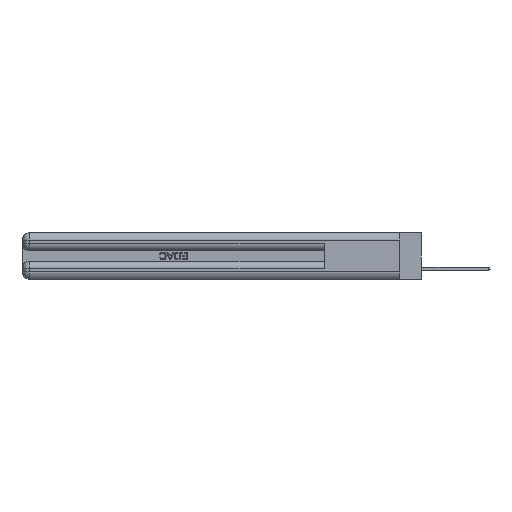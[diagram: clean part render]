
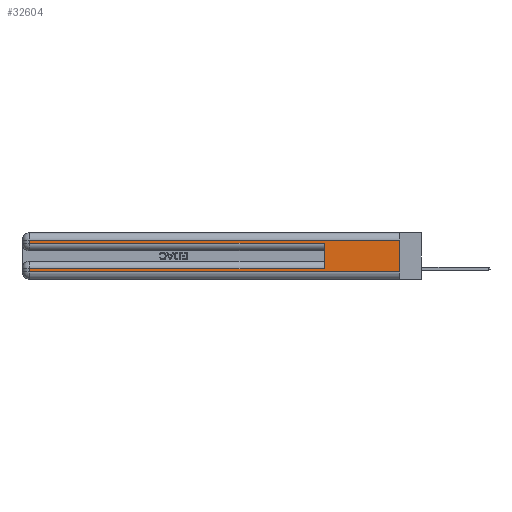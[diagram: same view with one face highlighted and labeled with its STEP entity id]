
A CAD part, left-side view. The second image highlights one B-rep face of the part: STEP entity #32604.
In plain terms, the highlighted planar face has unit normal (-1, 0, 0).
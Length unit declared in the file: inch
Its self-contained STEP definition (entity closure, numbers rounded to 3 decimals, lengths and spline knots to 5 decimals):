
#345 = ORIENTED_EDGE ( 'NONE', *, *, #15838, .F. ) ;
#2131 = CARTESIAN_POINT ( 'NONE',  ( 0., 0., 0.31 ) ) ;
#2187 = DIRECTION ( 'NONE',  ( 0., 0., 1. ) ) ;
#2577 = LINE ( 'NONE', #20068, #21641 ) ;
#3055 = VECTOR ( 'NONE', #5408, 39.37008 ) ;
#3238 = VECTOR ( 'NONE', #14824, 39.37008 ) ;
#3482 = EDGE_CURVE ( 'NONE', #24509, #18671, #12868, .T. ) ;
#3829 = LINE ( 'NONE', #23897, #10947 ) ;
#4015 = DIRECTION ( 'NONE',  ( 0., 0., -1. ) ) ;
#5408 = DIRECTION ( 'NONE',  ( 0., -1., 0. ) ) ;
#6729 = AXIS2_PLACEMENT_3D ( 'NONE', #31331, #17486, #4015 ) ;
#7187 = VERTEX_POINT ( 'NONE', #2131 ) ;
#7640 = CARTESIAN_POINT ( 'NONE',  ( 0., 2.94, 0.31 ) ) ;
#7705 = CARTESIAN_POINT ( 'NONE',  ( 0., 0., 0.085 ) ) ;
#7799 = ORIENTED_EDGE ( 'NONE', *, *, #21911, .F. ) ;
#8224 = CARTESIAN_POINT ( 'NONE',  ( 0., 0., 0.31 ) ) ;
#8374 = VECTOR ( 'NONE', #11844, 39.37008 ) ;
#8451 = EDGE_CURVE ( 'NONE', #42391, #24509, #31142, .T. ) ;
#8482 = DIRECTION ( 'NONE',  ( 0., 1., 0. ) ) ;
#8803 = EDGE_CURVE ( 'NONE', #11566, #16770, #3829, .T. ) ;
#9508 = LINE ( 'NONE', #8224, #8374 ) ;
#10862 = LINE ( 'NONE', #22340, #3238 ) ;
#10947 = VECTOR ( 'NONE', #34876, 39.37008 ) ;
#11481 = VECTOR ( 'NONE', #19316, 39.37008 ) ;
#11566 = VERTEX_POINT ( 'NONE', #7640 ) ;
#11844 = DIRECTION ( 'NONE',  ( 0., 1., 0. ) ) ;
#12608 = ORIENTED_EDGE ( 'NONE', *, *, #8803, .T. ) ;
#12868 = LINE ( 'NONE', #26767, #3055 ) ;
#13371 = VECTOR ( 'NONE', #2187, 39.37008 ) ;
#13522 = ORIENTED_EDGE ( 'NONE', *, *, #26812, .T. ) ;
#14137 = PLANE ( 'NONE',  #6729 ) ;
#14147 = ORIENTED_EDGE ( 'NONE', *, *, #20639, .T. ) ;
#14597 = CARTESIAN_POINT ( 'NONE',  ( 0., 0., 0.06 ) ) ;
#14824 = DIRECTION ( 'NONE',  ( 0., -1., 0. ) ) ;
#15838 = EDGE_CURVE ( 'NONE', #18775, #34628, #32902, .T. ) ;
#16158 = ORIENTED_EDGE ( 'NONE', *, *, #8451, .T. ) ;
#16770 = VERTEX_POINT ( 'NONE', #20675 ) ;
#17486 = DIRECTION ( 'NONE',  ( 1., 0., 0. ) ) ;
#17708 = CARTESIAN_POINT ( 'NONE',  ( 0., 0.6, 0.285 ) ) ;
#18671 = VERTEX_POINT ( 'NONE', #14597 ) ;
#18775 = VERTEX_POINT ( 'NONE', #37422 ) ;
#19316 = DIRECTION ( 'NONE',  ( 0., 0., -1. ) ) ;
#20068 = CARTESIAN_POINT ( 'NONE',  ( 0., 0., 0.37 ) ) ;
#20639 = EDGE_CURVE ( 'NONE', #16770, #34628, #10862, .T. ) ;
#20675 = CARTESIAN_POINT ( 'NONE',  ( 0., 2.94, 0.285 ) ) ;
#20952 = FACE_OUTER_BOUND ( 'NONE', #38707, .T. ) ;
#21641 = VECTOR ( 'NONE', #44315, 39.37008 ) ;
#21911 = EDGE_CURVE ( 'NONE', #7187, #18671, #2577, .T. ) ;
#22340 = CARTESIAN_POINT ( 'NONE',  ( 0., 0., 0.285 ) ) ;
#22583 = ORIENTED_EDGE ( 'NONE', *, *, #3482, .T. ) ;
#22791 = EDGE_CURVE ( 'NONE', #7187, #11566, #9508, .T. ) ;
#23897 = CARTESIAN_POINT ( 'NONE',  ( 0., 2.94, 0.37 ) ) ;
#24509 = VERTEX_POINT ( 'NONE', #39832 ) ;
#26767 = CARTESIAN_POINT ( 'NONE',  ( 0., 0., 0.06 ) ) ;
#26812 = EDGE_CURVE ( 'NONE', #18775, #42391, #39499, .T. ) ;
#29696 = CARTESIAN_POINT ( 'NONE',  ( 0., 2.94, 0.37 ) ) ;
#30372 = VECTOR ( 'NONE', #8482, 39.37008 ) ;
#31142 = LINE ( 'NONE', #29696, #11481 ) ;
#31331 = CARTESIAN_POINT ( 'NONE',  ( 0., 0., 0.37 ) ) ;
#32604 = ADVANCED_FACE ( 'NONE', ( #20952 ), #14137, .F. ) ;
#32902 = LINE ( 'NONE', #42262, #13371 ) ;
#34628 = VERTEX_POINT ( 'NONE', #17708 ) ;
#34876 = DIRECTION ( 'NONE',  ( 0., 0., -1. ) ) ;
#37422 = CARTESIAN_POINT ( 'NONE',  ( 0., 0.6, 0.085 ) ) ;
#38707 = EDGE_LOOP ( 'NONE', ( #7799, #42990, #12608, #14147, #345, #13522, #16158, #22583 ) ) ;
#39499 = LINE ( 'NONE', #7705, #30372 ) ;
#39832 = CARTESIAN_POINT ( 'NONE',  ( 0., 2.94, 0.06 ) ) ;
#41889 = CARTESIAN_POINT ( 'NONE',  ( 0., 2.94, 0.085 ) ) ;
#42262 = CARTESIAN_POINT ( 'NONE',  ( 0., 0.6, 0.145 ) ) ;
#42391 = VERTEX_POINT ( 'NONE', #41889 ) ;
#42990 = ORIENTED_EDGE ( 'NONE', *, *, #22791, .T. ) ;
#44315 = DIRECTION ( 'NONE',  ( 0., 0., -1. ) ) ;
